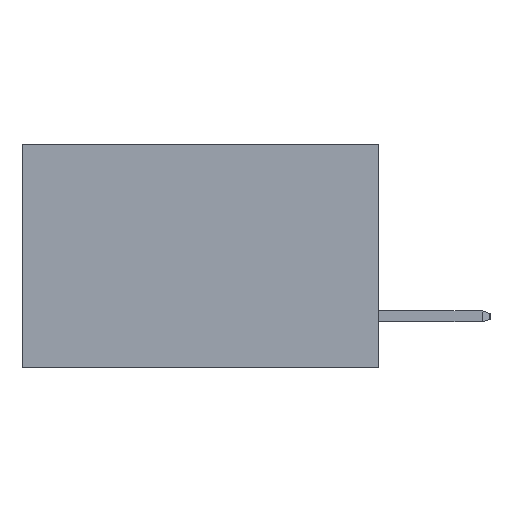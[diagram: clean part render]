
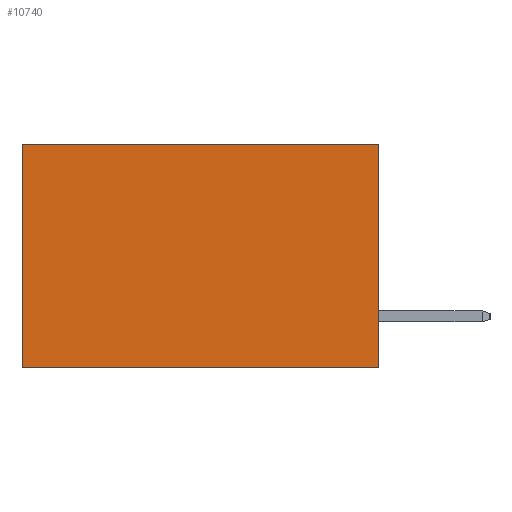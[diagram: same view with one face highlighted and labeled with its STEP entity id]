
A CAD part, left-side view. The second image highlights one B-rep face of the part: STEP entity #10740.
In plain terms, the highlighted planar face has unit normal (-1, 0, 0).
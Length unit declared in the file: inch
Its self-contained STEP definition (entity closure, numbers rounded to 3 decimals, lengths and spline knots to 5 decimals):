
#132 = ORIENTED_EDGE ( 'NONE', *, *, #11398, .T. ) ;
#695 = CARTESIAN_POINT ( 'NONE',  ( 0.277, 0.59, -0.37 ) ) ;
#1360 = DIRECTION ( 'NONE',  ( 0., 0., -1. ) ) ;
#1397 = VECTOR ( 'NONE', #9840, 39.37008 ) ;
#1979 = EDGE_LOOP ( 'NONE', ( #132, #6477, #3904, #6058 ) ) ;
#2496 = VECTOR ( 'NONE', #11331, 39.37008 ) ;
#2534 = CARTESIAN_POINT ( 'NONE',  ( 0.277, 0., -0.37 ) ) ;
#3793 = CARTESIAN_POINT ( 'NONE',  ( 0.277, 0.59, 0. ) ) ;
#3904 = ORIENTED_EDGE ( 'NONE', *, *, #9442, .F. ) ;
#4298 = VERTEX_POINT ( 'NONE', #5333 ) ;
#4791 = CARTESIAN_POINT ( 'NONE',  ( 0.277, 0., -0.37 ) ) ;
#5020 = VERTEX_POINT ( 'NONE', #8812 ) ;
#5333 = CARTESIAN_POINT ( 'NONE',  ( 0.277, 0., 0. ) ) ;
#5378 = VERTEX_POINT ( 'NONE', #7673 ) ;
#5755 = DIRECTION ( 'NONE',  ( 0., 0., -1. ) ) ;
#6058 = ORIENTED_EDGE ( 'NONE', *, *, #11570, .T. ) ;
#6084 = LINE ( 'NONE', #2534, #10997 ) ;
#6477 = ORIENTED_EDGE ( 'NONE', *, *, #7041, .F. ) ;
#7041 = EDGE_CURVE ( 'NONE', #5378, #5020, #10294, .T. ) ;
#7673 = CARTESIAN_POINT ( 'NONE',  ( 0.277, 0., -0.37 ) ) ;
#8438 = VECTOR ( 'NONE', #8571, 39.37008 ) ;
#8571 = DIRECTION ( 'NONE',  ( 0., 0., -1. ) ) ;
#8603 = FACE_OUTER_BOUND ( 'NONE', #1979, .T. ) ;
#8746 = LINE ( 'NONE', #695, #8438 ) ;
#8812 = CARTESIAN_POINT ( 'NONE',  ( 0.277, 0.59, -0.37 ) ) ;
#8839 = CARTESIAN_POINT ( 'NONE',  ( 0.277, 0., 0. ) ) ;
#9220 = LINE ( 'NONE', #8839, #1397 ) ;
#9442 = EDGE_CURVE ( 'NONE', #4298, #5378, #6084, .T. ) ;
#9840 = DIRECTION ( 'NONE',  ( 0., 1., 0. ) ) ;
#10294 = LINE ( 'NONE', #11559, #2496 ) ;
#10634 = PLANE ( 'NONE',  #12632 ) ;
#10740 = ADVANCED_FACE ( 'NONE', ( #8603 ), #10634, .F. ) ;
#10760 = VERTEX_POINT ( 'NONE', #3793 ) ;
#10997 = VECTOR ( 'NONE', #1360, 39.37008 ) ;
#11331 = DIRECTION ( 'NONE',  ( 0., 1., 0. ) ) ;
#11398 = EDGE_CURVE ( 'NONE', #10760, #5020, #8746, .T. ) ;
#11559 = CARTESIAN_POINT ( 'NONE',  ( 0.277, 0., -0.37 ) ) ;
#11570 = EDGE_CURVE ( 'NONE', #4298, #10760, #9220, .T. ) ;
#11651 = DIRECTION ( 'NONE',  ( 1., 0., 0. ) ) ;
#12632 = AXIS2_PLACEMENT_3D ( 'NONE', #4791, #11651, #5755 ) ;
